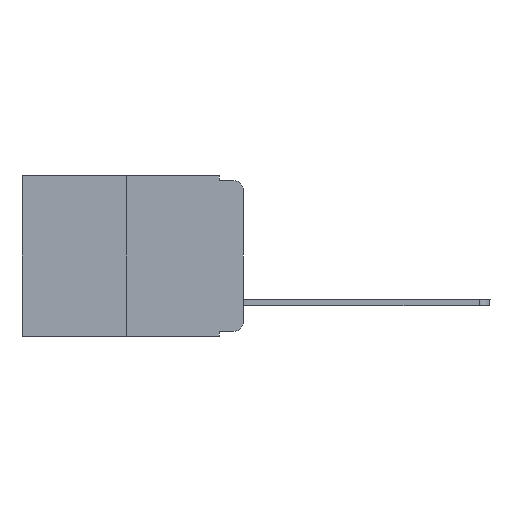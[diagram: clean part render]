
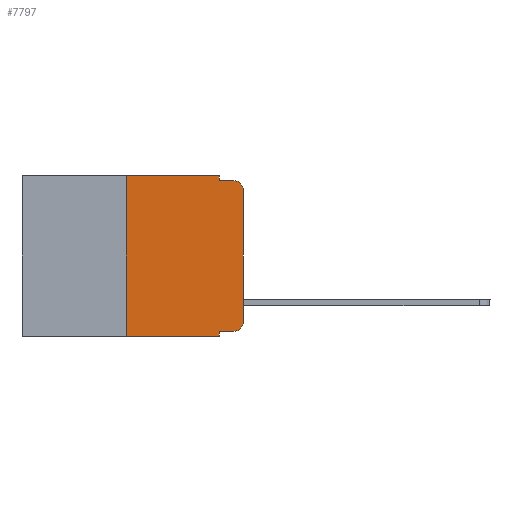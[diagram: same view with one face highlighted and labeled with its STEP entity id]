
A CAD part, left-side view. The second image highlights one B-rep face of the part: STEP entity #7797.
In plain terms, the highlighted planar face has unit normal (-1, 0, 0).
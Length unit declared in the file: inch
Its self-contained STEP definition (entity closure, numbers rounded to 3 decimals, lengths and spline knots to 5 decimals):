
#15 = LINE ( 'NONE', #5365, #4399 ) ;
#103 = ORIENTED_EDGE ( 'NONE', *, *, #3412, .F. ) ;
#275 = DIRECTION ( 'NONE',  ( 1., 0., 0. ) ) ;
#412 = VERTEX_POINT ( 'NONE', #1184 ) ;
#474 = EDGE_CURVE ( 'NONE', #9477, #412, #627, .T. ) ;
#627 = LINE ( 'NONE', #4895, #4665 ) ;
#803 = DIRECTION ( 'NONE',  ( 0., 0., 1. ) ) ;
#1028 = AXIS2_PLACEMENT_3D ( 'NONE', #1070, #275, #7889 ) ;
#1035 = LINE ( 'NONE', #5355, #8438 ) ;
#1070 = CARTESIAN_POINT ( 'NONE',  ( 0., 0.473, 0. ) ) ;
#1184 = CARTESIAN_POINT ( 'NONE',  ( 0., 0.02, -0.01 ) ) ;
#1249 = VECTOR ( 'NONE', #8171, 39.37008 ) ;
#1258 = VECTOR ( 'NONE', #11011, 39.37008 ) ;
#1352 = AXIS2_PLACEMENT_3D ( 'NONE', #5897, #9256, #9097 ) ;
#1385 = VECTOR ( 'NONE', #5722, 39.37008 ) ;
#1397 = CARTESIAN_POINT ( 'NONE',  ( 0., 0.051, -0.333 ) ) ;
#1702 = EDGE_CURVE ( 'NONE', #6430, #10873, #7702, .T. ) ;
#1960 = EDGE_CURVE ( 'NONE', #5182, #4310, #8393, .T. ) ;
#1972 = CARTESIAN_POINT ( 'NONE',  ( 0., 0.051, -0.343 ) ) ;
#2109 = CARTESIAN_POINT ( 'NONE',  ( 0., 0.051, 0. ) ) ;
#2688 = CARTESIAN_POINT ( 'NONE',  ( 0., 0.051, 0. ) ) ;
#2877 = CARTESIAN_POINT ( 'NONE',  ( 0., 0.02, -0.333 ) ) ;
#2920 = CARTESIAN_POINT ( 'NONE',  ( 0., 0.02, -0.313 ) ) ;
#3412 = EDGE_CURVE ( 'NONE', #4310, #8829, #1035, .T. ) ;
#3428 = EDGE_LOOP ( 'NONE', ( #9388, #5519, #6054, #4496, #103, #4919, #8882, #5821, #8280, #5003 ) ) ;
#3477 = LINE ( 'NONE', #2688, #8454 ) ;
#3650 = VERTEX_POINT ( 'NONE', #7664 ) ;
#3688 = VERTEX_POINT ( 'NONE', #10467 ) ;
#3734 = PLANE ( 'NONE',  #1028 ) ;
#3972 = EDGE_CURVE ( 'NONE', #8829, #9477, #3477, .T. ) ;
#4211 = CARTESIAN_POINT ( 'NONE',  ( 0., 0.051, -0.01 ) ) ;
#4251 = CIRCLE ( 'NONE', #8148, 0.02 ) ;
#4310 = VERTEX_POINT ( 'NONE', #9841 ) ;
#4357 = DIRECTION ( 'NONE',  ( 0., 0., -1. ) ) ;
#4399 = VECTOR ( 'NONE', #6135, 39.37008 ) ;
#4496 = ORIENTED_EDGE ( 'NONE', *, *, #3972, .F. ) ;
#4665 = VECTOR ( 'NONE', #7300, 39.37008 ) ;
#4784 = LINE ( 'NONE', #10439, #1249 ) ;
#4895 = CARTESIAN_POINT ( 'NONE',  ( 0., 0.051, -0.01 ) ) ;
#4919 = ORIENTED_EDGE ( 'NONE', *, *, #1960, .F. ) ;
#5003 = ORIENTED_EDGE ( 'NONE', *, *, #5022, .T. ) ;
#5022 = EDGE_CURVE ( 'NONE', #6254, #3650, #4251, .T. ) ;
#5182 = VERTEX_POINT ( 'NONE', #8365 ) ;
#5355 = CARTESIAN_POINT ( 'NONE',  ( 0., 0.473, 0. ) ) ;
#5365 = CARTESIAN_POINT ( 'NONE',  ( 0., 0.051, -0.333 ) ) ;
#5405 = VECTOR ( 'NONE', #803, 39.37008 ) ;
#5519 = ORIENTED_EDGE ( 'NONE', *, *, #9325, .T. ) ;
#5722 = DIRECTION ( 'NONE',  ( 0., 0., 1. ) ) ;
#5821 = ORIENTED_EDGE ( 'NONE', *, *, #1702, .F. ) ;
#5897 = CARTESIAN_POINT ( 'NONE',  ( 0., 0.02, -0.03 ) ) ;
#6054 = ORIENTED_EDGE ( 'NONE', *, *, #474, .F. ) ;
#6135 = DIRECTION ( 'NONE',  ( 0., -1., 0. ) ) ;
#6254 = VERTEX_POINT ( 'NONE', #2877 ) ;
#6430 = VERTEX_POINT ( 'NONE', #1397 ) ;
#6618 = EDGE_CURVE ( 'NONE', #6430, #6254, #15, .T. ) ;
#6686 = CARTESIAN_POINT ( 'NONE',  ( 0., 0.25, 0. ) ) ;
#7184 = EDGE_CURVE ( 'NONE', #5182, #10873, #4784, .T. ) ;
#7300 = DIRECTION ( 'NONE',  ( 0., -1., 0. ) ) ;
#7326 = DIRECTION ( 'NONE',  ( -1., 0., 0. ) ) ;
#7664 = CARTESIAN_POINT ( 'NONE',  ( 0., 0., -0.313 ) ) ;
#7702 = LINE ( 'NONE', #2109, #1258 ) ;
#7797 = ADVANCED_FACE ( 'NONE', ( #8202 ), #3734, .F. ) ;
#7819 = EDGE_CURVE ( 'NONE', #3650, #3688, #9085, .T. ) ;
#7889 = DIRECTION ( 'NONE',  ( 0., 0., -1. ) ) ;
#7949 = CARTESIAN_POINT ( 'NONE',  ( 0., 0., 0. ) ) ;
#7981 = DIRECTION ( 'NONE',  ( 0., 0., -1. ) ) ;
#8148 = AXIS2_PLACEMENT_3D ( 'NONE', #2920, #7326, #7981 ) ;
#8171 = DIRECTION ( 'NONE',  ( 0., -1., 0. ) ) ;
#8202 = FACE_OUTER_BOUND ( 'NONE', #3428, .T. ) ;
#8279 = CARTESIAN_POINT ( 'NONE',  ( 0., 0.051, 0. ) ) ;
#8280 = ORIENTED_EDGE ( 'NONE', *, *, #6618, .T. ) ;
#8365 = CARTESIAN_POINT ( 'NONE',  ( 0., 0.25, -0.343 ) ) ;
#8393 = LINE ( 'NONE', #6686, #5405 ) ;
#8438 = VECTOR ( 'NONE', #8733, 39.37008 ) ;
#8454 = VECTOR ( 'NONE', #4357, 39.37008 ) ;
#8733 = DIRECTION ( 'NONE',  ( 0., -1., 0. ) ) ;
#8829 = VERTEX_POINT ( 'NONE', #8279 ) ;
#8882 = ORIENTED_EDGE ( 'NONE', *, *, #7184, .T. ) ;
#9085 = LINE ( 'NONE', #7949, #1385 ) ;
#9097 = DIRECTION ( 'NONE',  ( 0., 0., -1. ) ) ;
#9256 = DIRECTION ( 'NONE',  ( -1., 0., 0. ) ) ;
#9325 = EDGE_CURVE ( 'NONE', #3688, #412, #10957, .T. ) ;
#9388 = ORIENTED_EDGE ( 'NONE', *, *, #7819, .T. ) ;
#9477 = VERTEX_POINT ( 'NONE', #4211 ) ;
#9841 = CARTESIAN_POINT ( 'NONE',  ( 0., 0.25, 0. ) ) ;
#10439 = CARTESIAN_POINT ( 'NONE',  ( 0., 0.473, -0.343 ) ) ;
#10467 = CARTESIAN_POINT ( 'NONE',  ( 0., 0., -0.03 ) ) ;
#10873 = VERTEX_POINT ( 'NONE', #1972 ) ;
#10957 = CIRCLE ( 'NONE', #1352, 0.02 ) ;
#11011 = DIRECTION ( 'NONE',  ( 0., 0., -1. ) ) ;
